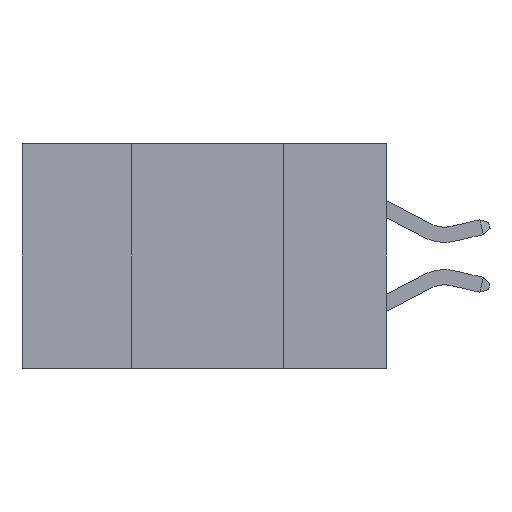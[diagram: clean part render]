
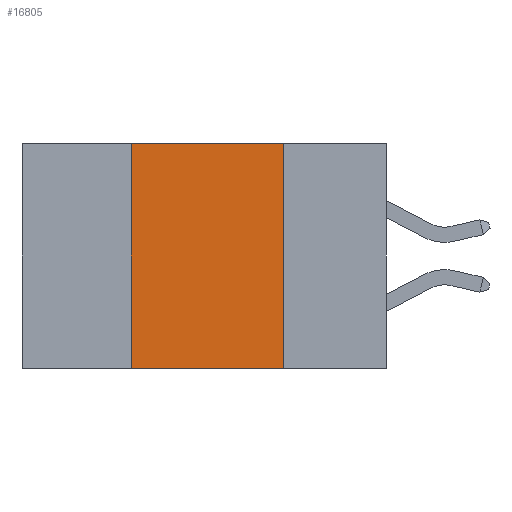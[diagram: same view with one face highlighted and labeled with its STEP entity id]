
A CAD part, left-side view. The second image highlights one B-rep face of the part: STEP entity #16805.
In plain terms, the highlighted planar face has unit normal (-1, 0, 0).
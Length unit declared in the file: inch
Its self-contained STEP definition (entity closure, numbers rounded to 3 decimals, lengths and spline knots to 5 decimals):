
#693 = AXIS2_PLACEMENT_3D ( 'NONE', #1063, #7150, #2320 ) ;
#1063 = CARTESIAN_POINT ( 'NONE',  ( 0., 0.6, 0. ) ) ;
#2320 = DIRECTION ( 'NONE',  ( 0., 0., -1. ) ) ;
#2577 = LINE ( 'NONE', #18727, #15967 ) ;
#2779 = VERTEX_POINT ( 'NONE', #20084 ) ;
#2945 = DIRECTION ( 'NONE',  ( 0., 0., -1. ) ) ;
#3399 = EDGE_LOOP ( 'NONE', ( #12704, #14373, #9340, #19234 ) ) ;
#5421 = VECTOR ( 'NONE', #2945, 39.37008 ) ;
#5495 = VERTEX_POINT ( 'NONE', #17121 ) ;
#5965 = CARTESIAN_POINT ( 'NONE',  ( 0., 0.6, -0.37 ) ) ;
#7150 = DIRECTION ( 'NONE',  ( 1., 0., 0. ) ) ;
#8870 = DIRECTION ( 'NONE',  ( 0., -1., 0. ) ) ;
#9112 = DIRECTION ( 'NONE',  ( 0., -1., 0. ) ) ;
#9340 = ORIENTED_EDGE ( 'NONE', *, *, #11252, .F. ) ;
#9462 = LINE ( 'NONE', #17316, #5421 ) ;
#9557 = EDGE_CURVE ( 'NONE', #15538, #2779, #20315, .T. ) ;
#10560 = LINE ( 'NONE', #18726, #18386 ) ;
#11252 = EDGE_CURVE ( 'NONE', #15538, #19540, #2577, .T. ) ;
#12704 = ORIENTED_EDGE ( 'NONE', *, *, #16947, .F. ) ;
#13238 = CARTESIAN_POINT ( 'NONE',  ( 0., 0.42, 0. ) ) ;
#14373 = ORIENTED_EDGE ( 'NONE', *, *, #14478, .F. ) ;
#14478 = EDGE_CURVE ( 'NONE', #19540, #5495, #10560, .T. ) ;
#15454 = PLANE ( 'NONE',  #693 ) ;
#15538 = VERTEX_POINT ( 'NONE', #20350 ) ;
#15967 = VECTOR ( 'NONE', #20294, 39.37008 ) ;
#15969 = VECTOR ( 'NONE', #9112, 39.37008 ) ;
#16697 = FACE_OUTER_BOUND ( 'NONE', #3399, .T. ) ;
#16805 = ADVANCED_FACE ( 'NONE', ( #16697 ), #15454, .F. ) ;
#16947 = EDGE_CURVE ( 'NONE', #5495, #2779, #9462, .T. ) ;
#17121 = CARTESIAN_POINT ( 'NONE',  ( 0., 0.17, 0. ) ) ;
#17316 = CARTESIAN_POINT ( 'NONE',  ( 0., 0.17, -0.37 ) ) ;
#18386 = VECTOR ( 'NONE', #8870, 39.37008 ) ;
#18726 = CARTESIAN_POINT ( 'NONE',  ( 0., 0.6, 0. ) ) ;
#18727 = CARTESIAN_POINT ( 'NONE',  ( 0., 0.42, -0.37 ) ) ;
#19234 = ORIENTED_EDGE ( 'NONE', *, *, #9557, .T. ) ;
#19540 = VERTEX_POINT ( 'NONE', #13238 ) ;
#20084 = CARTESIAN_POINT ( 'NONE',  ( 0., 0.17, -0.37 ) ) ;
#20294 = DIRECTION ( 'NONE',  ( 0., 0., 1. ) ) ;
#20315 = LINE ( 'NONE', #5965, #15969 ) ;
#20350 = CARTESIAN_POINT ( 'NONE',  ( 0., 0.42, -0.37 ) ) ;
